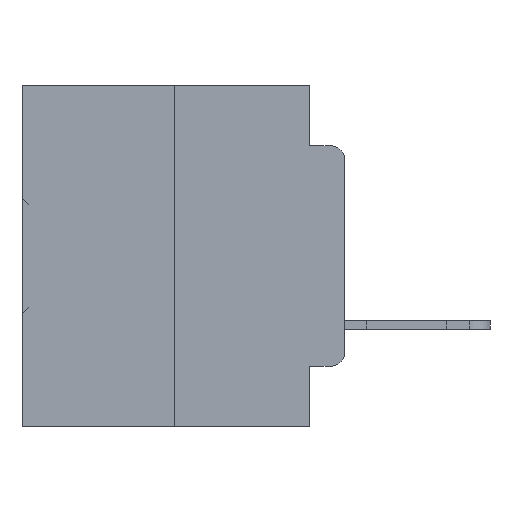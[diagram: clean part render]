
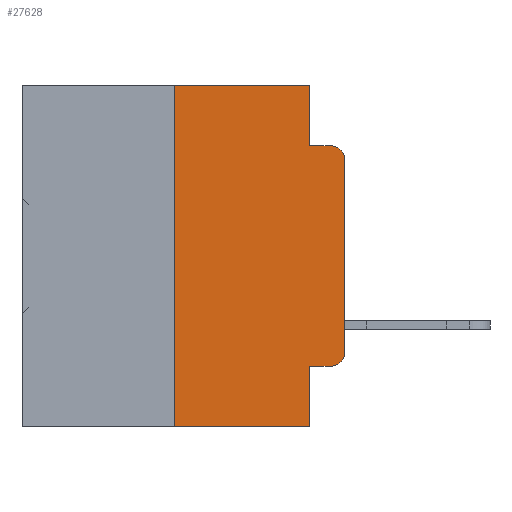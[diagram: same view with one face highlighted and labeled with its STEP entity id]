
A CAD part, left-side view. The second image highlights one B-rep face of the part: STEP entity #27628.
In plain terms, the highlighted planar face has unit normal (-1, 0, 0).
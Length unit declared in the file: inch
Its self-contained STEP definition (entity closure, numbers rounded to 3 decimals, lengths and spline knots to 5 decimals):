
#25 = EDGE_CURVE ( 'NONE', #10409, #23642, #10697, .T. ) ;
#572 = EDGE_CURVE ( 'NONE', #17168, #12281, #5236, .T. ) ;
#2122 = ORIENTED_EDGE ( 'NONE', *, *, #6643, .T. ) ;
#2653 = EDGE_CURVE ( 'NONE', #10409, #9868, #11820, .T. ) ;
#2864 = DIRECTION ( 'NONE',  ( 0., -1., 0. ) ) ;
#3689 = AXIS2_PLACEMENT_3D ( 'NONE', #35288, #35031, #34954 ) ;
#4112 = VECTOR ( 'NONE', #7119, 39.37008 ) ;
#4565 = VERTEX_POINT ( 'NONE', #6950 ) ;
#4644 = EDGE_CURVE ( 'NONE', #20469, #23642, #33278, .T. ) ;
#5236 = LINE ( 'NONE', #20755, #27116 ) ;
#5286 = CARTESIAN_POINT ( 'NONE',  ( 0., 0.02, -0.0885 ) ) ;
#6643 = EDGE_CURVE ( 'NONE', #20469, #17853, #33581, .T. ) ;
#6950 = CARTESIAN_POINT ( 'NONE',  ( 0., 0., -0.3915 ) ) ;
#7017 = CARTESIAN_POINT ( 'NONE',  ( 0., 0., -0.1085 ) ) ;
#7119 = DIRECTION ( 'NONE',  ( 0., 0., 1. ) ) ;
#7411 = ORIENTED_EDGE ( 'NONE', *, *, #30072, .T. ) ;
#8558 = EDGE_CURVE ( 'NONE', #17853, #4565, #13127, .T. ) ;
#9868 = VERTEX_POINT ( 'NONE', #20939 ) ;
#10409 = VERTEX_POINT ( 'NONE', #11387 ) ;
#10526 = VERTEX_POINT ( 'NONE', #5286 ) ;
#10697 = LINE ( 'NONE', #19049, #32098 ) ;
#10861 = DIRECTION ( 'NONE',  ( 0., 0., -1. ) ) ;
#11387 = CARTESIAN_POINT ( 'NONE',  ( 0., 0.25, -0.5 ) ) ;
#11522 = VECTOR ( 'NONE', #14579, 39.37008 ) ;
#11756 = PLANE ( 'NONE',  #11935 ) ;
#11820 = LINE ( 'NONE', #21747, #4112 ) ;
#11864 = CARTESIAN_POINT ( 'NONE',  ( 0., 0.473, 0. ) ) ;
#11935 = AXIS2_PLACEMENT_3D ( 'NONE', #11864, #31444, #14822 ) ;
#12013 = DIRECTION ( 'NONE',  ( -1., 0., 0. ) ) ;
#12094 = DIRECTION ( 'NONE',  ( 0., -1., 0. ) ) ;
#12281 = VERTEX_POINT ( 'NONE', #16365 ) ;
#12326 = VECTOR ( 'NONE', #2864, 39.37008 ) ;
#12334 = EDGE_LOOP ( 'NONE', ( #7411, #20577, #29551, #36430, #34573, #33845, #33731, #33026, #2122, #12637 ) ) ;
#12529 = DIRECTION ( 'NONE',  ( 0., -1., 0. ) ) ;
#12637 = ORIENTED_EDGE ( 'NONE', *, *, #8558, .T. ) ;
#13127 = CIRCLE ( 'NONE', #3689, 0.02 ) ;
#13643 = CARTESIAN_POINT ( 'NONE',  ( 0., 0., 0. ) ) ;
#14117 = EDGE_CURVE ( 'NONE', #9868, #17168, #19309, .T. ) ;
#14579 = DIRECTION ( 'NONE',  ( 0., -1., 0. ) ) ;
#14822 = DIRECTION ( 'NONE',  ( 0., 0., -1. ) ) ;
#15939 = CARTESIAN_POINT ( 'NONE',  ( 0., 0.473, 0. ) ) ;
#16208 = LINE ( 'NONE', #34142, #35362 ) ;
#16268 = CARTESIAN_POINT ( 'NONE',  ( 0., 0.02, -0.4115 ) ) ;
#16365 = CARTESIAN_POINT ( 'NONE',  ( 0., 0.051, -0.0885 ) ) ;
#16601 = DIRECTION ( 'NONE',  ( 0., 0., 1. ) ) ;
#16635 = CARTESIAN_POINT ( 'NONE',  ( 0., 0.051, 0. ) ) ;
#17168 = VERTEX_POINT ( 'NONE', #27610 ) ;
#17853 = VERTEX_POINT ( 'NONE', #16268 ) ;
#18852 = VECTOR ( 'NONE', #10861, 39.37008 ) ;
#19049 = CARTESIAN_POINT ( 'NONE',  ( 0., 0.473, -0.5 ) ) ;
#19309 = LINE ( 'NONE', #15939, #11522 ) ;
#20469 = VERTEX_POINT ( 'NONE', #29629 ) ;
#20577 = ORIENTED_EDGE ( 'NONE', *, *, #31795, .T. ) ;
#20755 = CARTESIAN_POINT ( 'NONE',  ( 0., 0.051, 0. ) ) ;
#20939 = CARTESIAN_POINT ( 'NONE',  ( 0., 0.25, 0. ) ) ;
#20962 = FACE_OUTER_BOUND ( 'NONE', #12334, .T. ) ;
#21101 = CARTESIAN_POINT ( 'NONE',  ( 0., 0.051, -0.4115 ) ) ;
#21747 = CARTESIAN_POINT ( 'NONE',  ( 0., 0.25, 0. ) ) ;
#22041 = CARTESIAN_POINT ( 'NONE',  ( 0., 0.051, -0.5 ) ) ;
#23642 = VERTEX_POINT ( 'NONE', #22041 ) ;
#27116 = VECTOR ( 'NONE', #30939, 39.37008 ) ;
#27610 = CARTESIAN_POINT ( 'NONE',  ( 0., 0.051, 0. ) ) ;
#27628 = ADVANCED_FACE ( 'NONE', ( #20962 ), #11756, .F. ) ;
#28961 = CARTESIAN_POINT ( 'NONE',  ( 0., 0.02, -0.1085 ) ) ;
#29551 = ORIENTED_EDGE ( 'NONE', *, *, #35282, .F. ) ;
#29629 = CARTESIAN_POINT ( 'NONE',  ( 0., 0.051, -0.4115 ) ) ;
#29994 = CIRCLE ( 'NONE', #33446, 0.02 ) ;
#30072 = EDGE_CURVE ( 'NONE', #4565, #31092, #32071, .T. ) ;
#30939 = DIRECTION ( 'NONE',  ( 0., 0., -1. ) ) ;
#31092 = VERTEX_POINT ( 'NONE', #7017 ) ;
#31277 = VECTOR ( 'NONE', #16601, 39.37008 ) ;
#31444 = DIRECTION ( 'NONE',  ( 1., 0., 0. ) ) ;
#31556 = DIRECTION ( 'NONE',  ( 0., 0., -1. ) ) ;
#31795 = EDGE_CURVE ( 'NONE', #31092, #10526, #29994, .T. ) ;
#32071 = LINE ( 'NONE', #13643, #31277 ) ;
#32098 = VECTOR ( 'NONE', #12529, 39.37008 ) ;
#33026 = ORIENTED_EDGE ( 'NONE', *, *, #4644, .F. ) ;
#33278 = LINE ( 'NONE', #16635, #18852 ) ;
#33446 = AXIS2_PLACEMENT_3D ( 'NONE', #28961, #12013, #31556 ) ;
#33581 = LINE ( 'NONE', #21101, #12326 ) ;
#33731 = ORIENTED_EDGE ( 'NONE', *, *, #25, .T. ) ;
#33845 = ORIENTED_EDGE ( 'NONE', *, *, #2653, .F. ) ;
#34142 = CARTESIAN_POINT ( 'NONE',  ( 0., 0.051, -0.0885 ) ) ;
#34573 = ORIENTED_EDGE ( 'NONE', *, *, #14117, .F. ) ;
#34954 = DIRECTION ( 'NONE',  ( 0., 0., -1. ) ) ;
#35031 = DIRECTION ( 'NONE',  ( -1., 0., 0. ) ) ;
#35282 = EDGE_CURVE ( 'NONE', #12281, #10526, #16208, .T. ) ;
#35288 = CARTESIAN_POINT ( 'NONE',  ( 0., 0.02, -0.3915 ) ) ;
#35362 = VECTOR ( 'NONE', #12094, 39.37008 ) ;
#36430 = ORIENTED_EDGE ( 'NONE', *, *, #572, .F. ) ;
